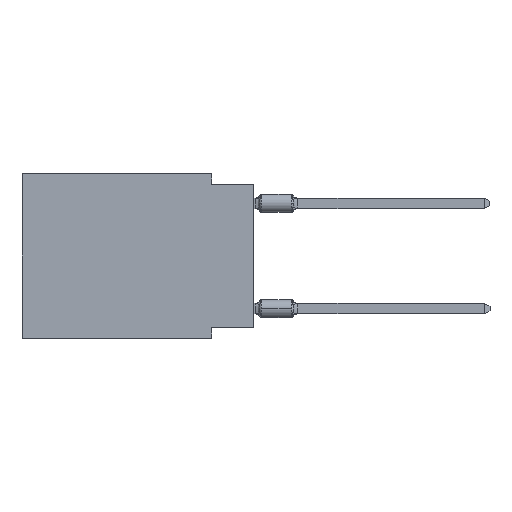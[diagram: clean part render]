
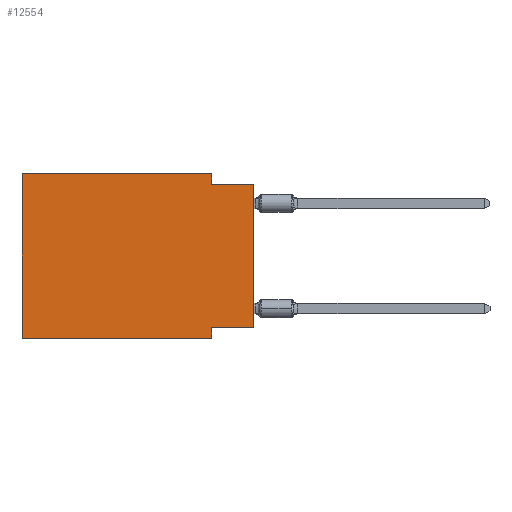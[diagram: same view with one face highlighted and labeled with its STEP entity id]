
A CAD part, left-side view. The second image highlights one B-rep face of the part: STEP entity #12554.
In plain terms, the highlighted planar face has unit normal (-1, 0, 0).
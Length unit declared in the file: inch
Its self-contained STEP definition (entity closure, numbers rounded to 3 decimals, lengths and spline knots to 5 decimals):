
#286 = DIRECTION ( 'NONE',  ( 0., -1., 0. ) ) ;
#303 = VERTEX_POINT ( 'NONE', #8339 ) ;
#1041 = LINE ( 'NONE', #8937, #8597 ) ;
#1309 = FACE_OUTER_BOUND ( 'NONE', #14836, .T. ) ;
#1904 = CARTESIAN_POINT ( 'NONE',  ( 0., 0., -0.365 ) ) ;
#1982 = DIRECTION ( 'NONE',  ( 0., -1., 0. ) ) ;
#2042 = EDGE_CURVE ( 'NONE', #21393, #8318, #3924, .T. ) ;
#2856 = ORIENTED_EDGE ( 'NONE', *, *, #5141, .F. ) ;
#3253 = LINE ( 'NONE', #13327, #4245 ) ;
#3582 = EDGE_CURVE ( 'NONE', #21809, #9002, #3253, .T. ) ;
#3924 = LINE ( 'NONE', #21628, #6680 ) ;
#4172 = CARTESIAN_POINT ( 'NONE',  ( 0., 0., -0.025 ) ) ;
#4245 = VECTOR ( 'NONE', #23294, 39.37008 ) ;
#4349 = EDGE_CURVE ( 'NONE', #21393, #6444, #17010, .T. ) ;
#4517 = DIRECTION ( 'NONE',  ( 0., 0., -1. ) ) ;
#4538 = DIRECTION ( 'NONE',  ( 0., -1., 0. ) ) ;
#4648 = CARTESIAN_POINT ( 'NONE',  ( 0., 0.1, -0.39 ) ) ;
#5130 = DIRECTION ( 'NONE',  ( 0., 0., 1. ) ) ;
#5139 = EDGE_CURVE ( 'NONE', #6444, #20254, #24193, .T. ) ;
#5141 = EDGE_CURVE ( 'NONE', #20254, #303, #1041, .T. ) ;
#5194 = CARTESIAN_POINT ( 'NONE',  ( 0., 0.55, 0. ) ) ;
#5723 = CARTESIAN_POINT ( 'NONE',  ( 0., 0.55, -0.39 ) ) ;
#6156 = DIRECTION ( 'NONE',  ( 0., 1., 0. ) ) ;
#6444 = VERTEX_POINT ( 'NONE', #16371 ) ;
#6680 = VECTOR ( 'NONE', #1982, 39.37008 ) ;
#8193 = VECTOR ( 'NONE', #4538, 39.37008 ) ;
#8318 = VERTEX_POINT ( 'NONE', #17622 ) ;
#8339 = CARTESIAN_POINT ( 'NONE',  ( 0., 0.1, -0.025 ) ) ;
#8597 = VECTOR ( 'NONE', #9180, 39.37008 ) ;
#8814 = ORIENTED_EDGE ( 'NONE', *, *, #5139, .F. ) ;
#8937 = CARTESIAN_POINT ( 'NONE',  ( 0., 0.1, 0. ) ) ;
#9002 = VERTEX_POINT ( 'NONE', #12295 ) ;
#9153 = ORIENTED_EDGE ( 'NONE', *, *, #4349, .F. ) ;
#9180 = DIRECTION ( 'NONE',  ( 0., 0., -1. ) ) ;
#9349 = ORIENTED_EDGE ( 'NONE', *, *, #18234, .F. ) ;
#10386 = CARTESIAN_POINT ( 'NONE',  ( 0., 0.1, -0.365 ) ) ;
#12295 = CARTESIAN_POINT ( 'NONE',  ( 0., 0., -0.025 ) ) ;
#12554 = ADVANCED_FACE ( 'NONE', ( #1309 ), #17579, .F. ) ;
#13327 = CARTESIAN_POINT ( 'NONE',  ( 0., 0., 0. ) ) ;
#13594 = EDGE_CURVE ( 'NONE', #21809, #22721, #17529, .T. ) ;
#13651 = ORIENTED_EDGE ( 'NONE', *, *, #3582, .T. ) ;
#14836 = EDGE_LOOP ( 'NONE', ( #13651, #21277, #2856, #8814, #9153, #24901, #9349, #24104 ) ) ;
#15746 = VECTOR ( 'NONE', #6156, 39.37008 ) ;
#16331 = CARTESIAN_POINT ( 'NONE',  ( 0., 0.1, 0. ) ) ;
#16371 = CARTESIAN_POINT ( 'NONE',  ( 0., 0.55, 0. ) ) ;
#17010 = LINE ( 'NONE', #25049, #19362 ) ;
#17529 = LINE ( 'NONE', #1904, #15746 ) ;
#17579 = PLANE ( 'NONE',  #21071 ) ;
#17622 = CARTESIAN_POINT ( 'NONE',  ( 0., 0.1, -0.39 ) ) ;
#17993 = LINE ( 'NONE', #4172, #20286 ) ;
#18234 = EDGE_CURVE ( 'NONE', #22721, #8318, #20018, .T. ) ;
#19362 = VECTOR ( 'NONE', #5130, 39.37008 ) ;
#20018 = LINE ( 'NONE', #4648, #25361 ) ;
#20254 = VERTEX_POINT ( 'NONE', #16331 ) ;
#20286 = VECTOR ( 'NONE', #286, 39.37008 ) ;
#21071 = AXIS2_PLACEMENT_3D ( 'NONE', #5194, #25496, #23284 ) ;
#21277 = ORIENTED_EDGE ( 'NONE', *, *, #22842, .F. ) ;
#21393 = VERTEX_POINT ( 'NONE', #5723 ) ;
#21628 = CARTESIAN_POINT ( 'NONE',  ( 0., 0.55, -0.39 ) ) ;
#21809 = VERTEX_POINT ( 'NONE', #25219 ) ;
#22721 = VERTEX_POINT ( 'NONE', #10386 ) ;
#22842 = EDGE_CURVE ( 'NONE', #303, #9002, #17993, .T. ) ;
#23284 = DIRECTION ( 'NONE',  ( 0., 0., -1. ) ) ;
#23294 = DIRECTION ( 'NONE',  ( 0., 0., 1. ) ) ;
#24104 = ORIENTED_EDGE ( 'NONE', *, *, #13594, .F. ) ;
#24193 = LINE ( 'NONE', #24451, #8193 ) ;
#24451 = CARTESIAN_POINT ( 'NONE',  ( 0., 0.55, 0. ) ) ;
#24901 = ORIENTED_EDGE ( 'NONE', *, *, #2042, .T. ) ;
#25049 = CARTESIAN_POINT ( 'NONE',  ( 0., 0.55, 0. ) ) ;
#25219 = CARTESIAN_POINT ( 'NONE',  ( 0., 0., -0.365 ) ) ;
#25361 = VECTOR ( 'NONE', #4517, 39.37008 ) ;
#25496 = DIRECTION ( 'NONE',  ( 1., 0., 0. ) ) ;
